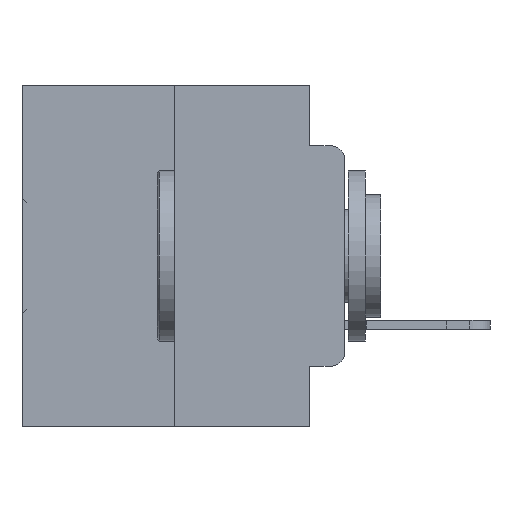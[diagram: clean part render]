
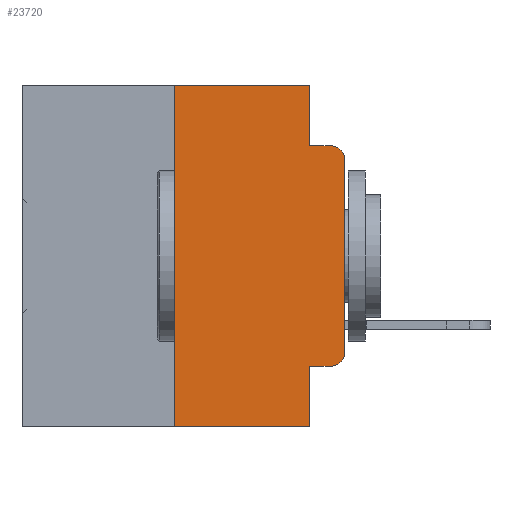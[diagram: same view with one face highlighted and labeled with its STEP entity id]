
A CAD part, left-side view. The second image highlights one B-rep face of the part: STEP entity #23720.
In plain terms, the highlighted planar face has unit normal (-1, 0, 0).
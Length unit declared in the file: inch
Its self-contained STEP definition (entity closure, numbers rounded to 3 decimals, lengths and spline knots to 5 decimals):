
#214 = EDGE_CURVE ( 'NONE', #30111, #5323, #32240, .T. ) ;
#632 = CARTESIAN_POINT ( 'NONE',  ( 0., 0.02, -0.3915 ) ) ;
#750 = DIRECTION ( 'NONE',  ( 0., 0., -1. ) ) ;
#1176 = VERTEX_POINT ( 'NONE', #21301 ) ;
#1473 = CARTESIAN_POINT ( 'NONE',  ( 0., 0.25, 0. ) ) ;
#1647 = CARTESIAN_POINT ( 'NONE',  ( 0., 0.051, -0.0885 ) ) ;
#1765 = ORIENTED_EDGE ( 'NONE', *, *, #11258, .T. ) ;
#2070 = DIRECTION ( 'NONE',  ( 0., -1., 0. ) ) ;
#2516 = VECTOR ( 'NONE', #4319, 39.37008 ) ;
#2647 = ORIENTED_EDGE ( 'NONE', *, *, #18864, .T. ) ;
#2682 = DIRECTION ( 'NONE',  ( 0., 0., -1. ) ) ;
#2900 = CARTESIAN_POINT ( 'NONE',  ( 0., 0., -0.3915 ) ) ;
#3133 = CARTESIAN_POINT ( 'NONE',  ( 0., 0.02, -0.0885 ) ) ;
#3420 = LINE ( 'NONE', #25551, #30512 ) ;
#3569 = DIRECTION ( 'NONE',  ( 0., 0., -1. ) ) ;
#3953 = ORIENTED_EDGE ( 'NONE', *, *, #23614, .T. ) ;
#4319 = DIRECTION ( 'NONE',  ( 0., 0., 1. ) ) ;
#5168 = AXIS2_PLACEMENT_3D ( 'NONE', #632, #19305, #3569 ) ;
#5213 = AXIS2_PLACEMENT_3D ( 'NONE', #22526, #7144, #24971 ) ;
#5323 = VERTEX_POINT ( 'NONE', #32546 ) ;
#5380 = VECTOR ( 'NONE', #7753, 39.37008 ) ;
#5585 = DIRECTION ( 'NONE',  ( 0., -1., 0. ) ) ;
#5668 = CIRCLE ( 'NONE', #5168, 0.02 ) ;
#5740 = VERTEX_POINT ( 'NONE', #21778 ) ;
#5959 = EDGE_CURVE ( 'NONE', #5323, #16003, #17747, .T. ) ;
#7144 = DIRECTION ( 'NONE',  ( -1., 0., 0. ) ) ;
#7433 = VECTOR ( 'NONE', #750, 39.37008 ) ;
#7722 = VECTOR ( 'NONE', #11390, 39.37008 ) ;
#7753 = DIRECTION ( 'NONE',  ( 0., 0., -1. ) ) ;
#8130 = FACE_OUTER_BOUND ( 'NONE', #13291, .T. ) ;
#8278 = LINE ( 'NONE', #31549, #7433 ) ;
#8830 = CARTESIAN_POINT ( 'NONE',  ( 0., 0., 0. ) ) ;
#9274 = VERTEX_POINT ( 'NONE', #31030 ) ;
#9567 = EDGE_CURVE ( 'NONE', #9732, #16003, #14614, .T. ) ;
#9732 = VERTEX_POINT ( 'NONE', #30456 ) ;
#10012 = ORIENTED_EDGE ( 'NONE', *, *, #31935, .F. ) ;
#10146 = VECTOR ( 'NONE', #5585, 39.37008 ) ;
#10754 = PLANE ( 'NONE',  #17953 ) ;
#10826 = CARTESIAN_POINT ( 'NONE',  ( 0., 0.473, 0. ) ) ;
#11258 = EDGE_CURVE ( 'NONE', #25514, #9732, #21426, .T. ) ;
#11386 = CARTESIAN_POINT ( 'NONE',  ( 0., 0.051, -0.5 ) ) ;
#11390 = DIRECTION ( 'NONE',  ( 0., 0., 1. ) ) ;
#11619 = DIRECTION ( 'NONE',  ( 0., -1., 0. ) ) ;
#12237 = LINE ( 'NONE', #26599, #24112 ) ;
#13291 = EDGE_LOOP ( 'NONE', ( #1765, #23078, #23468, #28809, #28449, #10012, #3953, #27637, #2647, #19212 ) ) ;
#14614 = CIRCLE ( 'NONE', #5213, 0.02 ) ;
#16003 = VERTEX_POINT ( 'NONE', #3133 ) ;
#16948 = VECTOR ( 'NONE', #2070, 39.37008 ) ;
#17053 = LINE ( 'NONE', #10826, #10146 ) ;
#17175 = EDGE_CURVE ( 'NONE', #9274, #25514, #5668, .T. ) ;
#17522 = CARTESIAN_POINT ( 'NONE',  ( 0., 0.25, 0. ) ) ;
#17747 = LINE ( 'NONE', #1647, #16948 ) ;
#17953 = AXIS2_PLACEMENT_3D ( 'NONE', #23407, #18573, #2682 ) ;
#18573 = DIRECTION ( 'NONE',  ( 1., 0., 0. ) ) ;
#18864 = EDGE_CURVE ( 'NONE', #1176, #9274, #12237, .T. ) ;
#19212 = ORIENTED_EDGE ( 'NONE', *, *, #17175, .T. ) ;
#19305 = DIRECTION ( 'NONE',  ( -1., 0., 0. ) ) ;
#19875 = CARTESIAN_POINT ( 'NONE',  ( 0., 0.051, 0. ) ) ;
#20283 = CARTESIAN_POINT ( 'NONE',  ( 0., 0.051, 0. ) ) ;
#21301 = CARTESIAN_POINT ( 'NONE',  ( 0., 0.051, -0.4115 ) ) ;
#21426 = LINE ( 'NONE', #8830, #7722 ) ;
#21778 = CARTESIAN_POINT ( 'NONE',  ( 0., 0.25, -0.5 ) ) ;
#22526 = CARTESIAN_POINT ( 'NONE',  ( 0., 0.02, -0.1085 ) ) ;
#23078 = ORIENTED_EDGE ( 'NONE', *, *, #9567, .T. ) ;
#23407 = CARTESIAN_POINT ( 'NONE',  ( 0., 0.473, 0. ) ) ;
#23468 = ORIENTED_EDGE ( 'NONE', *, *, #5959, .F. ) ;
#23614 = EDGE_CURVE ( 'NONE', #5740, #27585, #3420, .T. ) ;
#23720 = ADVANCED_FACE ( 'NONE', ( #8130 ), #10754, .F. ) ;
#24112 = VECTOR ( 'NONE', #11619, 39.37008 ) ;
#24458 = EDGE_CURVE ( 'NONE', #28872, #30111, #17053, .T. ) ;
#24971 = DIRECTION ( 'NONE',  ( 0., 0., -1. ) ) ;
#25514 = VERTEX_POINT ( 'NONE', #2900 ) ;
#25551 = CARTESIAN_POINT ( 'NONE',  ( 0., 0.473, -0.5 ) ) ;
#26599 = CARTESIAN_POINT ( 'NONE',  ( 0., 0.051, -0.4115 ) ) ;
#27585 = VERTEX_POINT ( 'NONE', #11386 ) ;
#27637 = ORIENTED_EDGE ( 'NONE', *, *, #28687, .F. ) ;
#28022 = DIRECTION ( 'NONE',  ( 0., -1., 0. ) ) ;
#28449 = ORIENTED_EDGE ( 'NONE', *, *, #24458, .F. ) ;
#28687 = EDGE_CURVE ( 'NONE', #1176, #27585, #8278, .T. ) ;
#28809 = ORIENTED_EDGE ( 'NONE', *, *, #214, .F. ) ;
#28872 = VERTEX_POINT ( 'NONE', #17522 ) ;
#29777 = LINE ( 'NONE', #1473, #2516 ) ;
#30111 = VERTEX_POINT ( 'NONE', #19875 ) ;
#30456 = CARTESIAN_POINT ( 'NONE',  ( 0., 0., -0.1085 ) ) ;
#30512 = VECTOR ( 'NONE', #28022, 39.37008 ) ;
#31030 = CARTESIAN_POINT ( 'NONE',  ( 0., 0.02, -0.4115 ) ) ;
#31549 = CARTESIAN_POINT ( 'NONE',  ( 0., 0.051, 0. ) ) ;
#31935 = EDGE_CURVE ( 'NONE', #5740, #28872, #29777, .T. ) ;
#32240 = LINE ( 'NONE', #20283, #5380 ) ;
#32546 = CARTESIAN_POINT ( 'NONE',  ( 0., 0.051, -0.0885 ) ) ;
